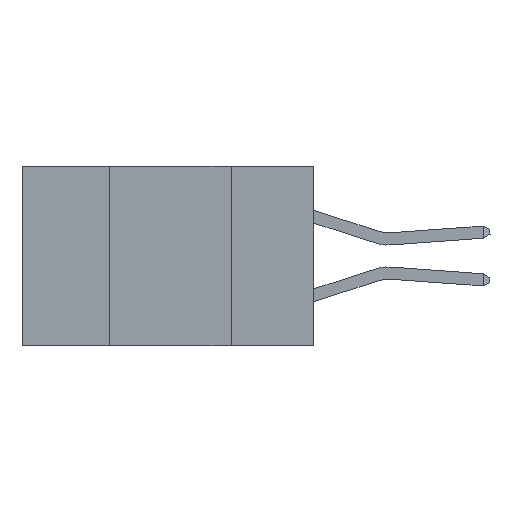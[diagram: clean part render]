
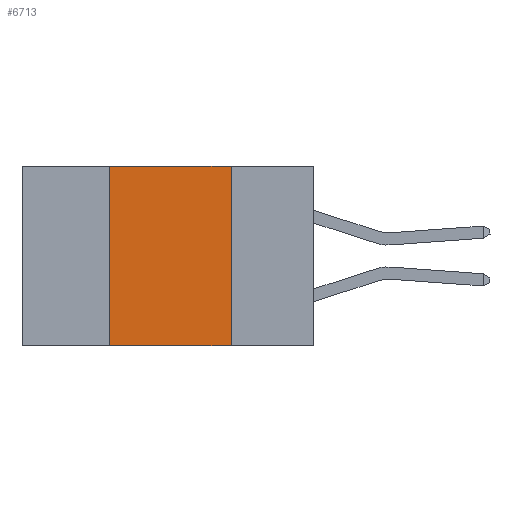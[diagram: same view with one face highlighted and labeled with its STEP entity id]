
A CAD part, left-side view. The second image highlights one B-rep face of the part: STEP entity #6713.
In plain terms, the highlighted planar face has unit normal (-1, 0, 0).
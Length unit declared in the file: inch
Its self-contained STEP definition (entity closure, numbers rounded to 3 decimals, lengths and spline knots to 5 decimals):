
#490 = LINE ( 'NONE', #1808, #3521 ) ;
#560 = DIRECTION ( 'NONE',  ( 0., -1., 0. ) ) ;
#577 = DIRECTION ( 'NONE',  ( 0., 0., 1. ) ) ;
#860 = LINE ( 'NONE', #10284, #14183 ) ;
#1808 = CARTESIAN_POINT ( 'NONE',  ( 0., 0.6, -0.37 ) ) ;
#2222 = ORIENTED_EDGE ( 'NONE', *, *, #4546, .F. ) ;
#2917 = CARTESIAN_POINT ( 'NONE',  ( 0., 0.17, 0. ) ) ;
#3002 = VECTOR ( 'NONE', #577, 39.37008 ) ;
#3521 = VECTOR ( 'NONE', #560, 39.37008 ) ;
#3801 = EDGE_CURVE ( 'NONE', #9805, #12886, #860, .T. ) ;
#4546 = EDGE_CURVE ( 'NONE', #7639, #9582, #11330, .T. ) ;
#4960 = EDGE_CURVE ( 'NONE', #7639, #12886, #490, .T. ) ;
#5826 = DIRECTION ( 'NONE',  ( 0., -1., 0. ) ) ;
#6713 = ADVANCED_FACE ( 'NONE', ( #13790 ), #7994, .F. ) ;
#7016 = CARTESIAN_POINT ( 'NONE',  ( 0., 0.17, -0.37 ) ) ;
#7050 = ORIENTED_EDGE ( 'NONE', *, *, #4960, .T. ) ;
#7639 = VERTEX_POINT ( 'NONE', #12659 ) ;
#7994 = PLANE ( 'NONE',  #10694 ) ;
#8042 = EDGE_LOOP ( 'NONE', ( #10928, #11577, #2222, #7050 ) ) ;
#8976 = DIRECTION ( 'NONE',  ( 0., 0., -1. ) ) ;
#9253 = DIRECTION ( 'NONE',  ( 0., 0., -1. ) ) ;
#9582 = VERTEX_POINT ( 'NONE', #11091 ) ;
#9805 = VERTEX_POINT ( 'NONE', #2917 ) ;
#10284 = CARTESIAN_POINT ( 'NONE',  ( 0., 0.17, 0. ) ) ;
#10416 = CARTESIAN_POINT ( 'NONE',  ( 0., 0.6, 0. ) ) ;
#10694 = AXIS2_PLACEMENT_3D ( 'NONE', #10416, #11603, #9253 ) ;
#10928 = ORIENTED_EDGE ( 'NONE', *, *, #3801, .F. ) ;
#11091 = CARTESIAN_POINT ( 'NONE',  ( 0., 0.42, 0. ) ) ;
#11105 = CARTESIAN_POINT ( 'NONE',  ( 0., 0.42, 0. ) ) ;
#11330 = LINE ( 'NONE', #11105, #3002 ) ;
#11577 = ORIENTED_EDGE ( 'NONE', *, *, #13426, .F. ) ;
#11603 = DIRECTION ( 'NONE',  ( 1., 0., 0. ) ) ;
#12659 = CARTESIAN_POINT ( 'NONE',  ( 0., 0.42, -0.37 ) ) ;
#12886 = VERTEX_POINT ( 'NONE', #7016 ) ;
#13426 = EDGE_CURVE ( 'NONE', #9582, #9805, #14024, .T. ) ;
#13580 = VECTOR ( 'NONE', #5826, 39.37008 ) ;
#13790 = FACE_OUTER_BOUND ( 'NONE', #8042, .T. ) ;
#14024 = LINE ( 'NONE', #15272, #13580 ) ;
#14183 = VECTOR ( 'NONE', #8976, 39.37008 ) ;
#15272 = CARTESIAN_POINT ( 'NONE',  ( 0., 0.6, 0. ) ) ;
